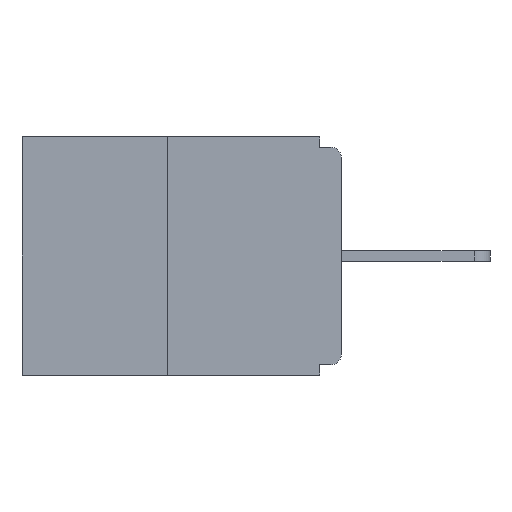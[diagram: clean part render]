
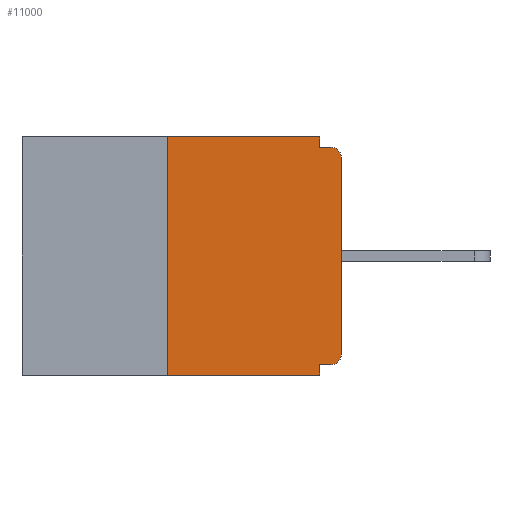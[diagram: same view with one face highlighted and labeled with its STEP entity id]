
A CAD part, left-side view. The second image highlights one B-rep face of the part: STEP entity #11000.
In plain terms, the highlighted planar face has unit normal (-1, 0, 0).
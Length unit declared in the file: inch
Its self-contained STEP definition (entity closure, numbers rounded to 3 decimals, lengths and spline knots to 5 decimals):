
#33 = ORIENTED_EDGE ( 'NONE', *, *, #8551, .F. ) ;
#312 = VERTEX_POINT ( 'NONE', #10353 ) ;
#502 = ORIENTED_EDGE ( 'NONE', *, *, #8499, .T. ) ;
#635 = CARTESIAN_POINT ( 'NONE',  ( 0., 0.031, 0. ) ) ;
#691 = ORIENTED_EDGE ( 'NONE', *, *, #5160, .F. ) ;
#935 = VERTEX_POINT ( 'NONE', #10460 ) ;
#1058 = VERTEX_POINT ( 'NONE', #6445 ) ;
#1236 = ORIENTED_EDGE ( 'NONE', *, *, #5236, .T. ) ;
#2130 = VECTOR ( 'NONE', #8110, 39.37008 ) ;
#2298 = CARTESIAN_POINT ( 'NONE',  ( 0., 0.25, 0. ) ) ;
#2444 = VERTEX_POINT ( 'NONE', #6638 ) ;
#2843 = CARTESIAN_POINT ( 'NONE',  ( 0., 0., -0.313 ) ) ;
#3059 = EDGE_LOOP ( 'NONE', ( #9164, #7493, #502, #33, #8696, #8607, #10615, #1236, #691, #9715 ) ) ;
#3133 = VERTEX_POINT ( 'NONE', #9784 ) ;
#3375 = FACE_OUTER_BOUND ( 'NONE', #3059, .T. ) ;
#3427 = VERTEX_POINT ( 'NONE', #2843 ) ;
#3431 = VERTEX_POINT ( 'NONE', #2298 ) ;
#3560 = EDGE_CURVE ( 'NONE', #3431, #7484, #9764, .T. ) ;
#3712 = LINE ( 'NONE', #10424, #4056 ) ;
#4029 = DIRECTION ( 'NONE',  ( 1., 0., 0. ) ) ;
#4056 = VECTOR ( 'NONE', #10441, 39.37008 ) ;
#4500 = VERTEX_POINT ( 'NONE', #4963 ) ;
#4961 = EDGE_CURVE ( 'NONE', #3427, #935, #11020, .T. ) ;
#4963 = CARTESIAN_POINT ( 'NONE',  ( 0., 0.25, -0.343 ) ) ;
#5100 = EDGE_CURVE ( 'NONE', #8013, #3133, #3712, .T. ) ;
#5160 = EDGE_CURVE ( 'NONE', #312, #1058, #5607, .T. ) ;
#5177 = EDGE_CURVE ( 'NONE', #8013, #3427, #7518, .T. ) ;
#5228 = VECTOR ( 'NONE', #8587, 39.37008 ) ;
#5236 = EDGE_CURVE ( 'NONE', #935, #1058, #7266, .T. ) ;
#5477 = LINE ( 'NONE', #8772, #5228 ) ;
#5510 = AXIS2_PLACEMENT_3D ( 'NONE', #7427, #4029, #9884 ) ;
#5607 = LINE ( 'NONE', #10196, #9704 ) ;
#5889 = CARTESIAN_POINT ( 'NONE',  ( 0., 0.015, -0.328 ) ) ;
#6445 = CARTESIAN_POINT ( 'NONE',  ( 0., 0.015, -0.015 ) ) ;
#6638 = CARTESIAN_POINT ( 'NONE',  ( 0., 0.031, -0.343 ) ) ;
#7266 = CIRCLE ( 'NONE', #10380, 0.015 ) ;
#7394 = VECTOR ( 'NONE', #8279, 39.37008 ) ;
#7427 = CARTESIAN_POINT ( 'NONE',  ( 0., 0.46, 0. ) ) ;
#7484 = VERTEX_POINT ( 'NONE', #635 ) ;
#7493 = ORIENTED_EDGE ( 'NONE', *, *, #8468, .F. ) ;
#7518 = CIRCLE ( 'NONE', #10393, 0.015 ) ;
#7664 = LINE ( 'NONE', #8174, #2130 ) ;
#7919 = LINE ( 'NONE', #9093, #11351 ) ;
#8013 = VERTEX_POINT ( 'NONE', #5889 ) ;
#8110 = DIRECTION ( 'NONE',  ( 0., 0., -1. ) ) ;
#8174 = CARTESIAN_POINT ( 'NONE',  ( 0., 0.031, 0. ) ) ;
#8259 = CARTESIAN_POINT ( 'NONE',  ( 0., 0.031, -0.343 ) ) ;
#8279 = DIRECTION ( 'NONE',  ( 0., 0., -1. ) ) ;
#8468 = EDGE_CURVE ( 'NONE', #4500, #3431, #7919, .T. ) ;
#8499 = EDGE_CURVE ( 'NONE', #4500, #2444, #5477, .T. ) ;
#8551 = EDGE_CURVE ( 'NONE', #3133, #2444, #9348, .T. ) ;
#8552 = EDGE_CURVE ( 'NONE', #7484, #312, #7664, .T. ) ;
#8587 = DIRECTION ( 'NONE',  ( 0., -1., 0. ) ) ;
#8607 = ORIENTED_EDGE ( 'NONE', *, *, #5177, .T. ) ;
#8696 = ORIENTED_EDGE ( 'NONE', *, *, #5100, .F. ) ;
#8772 = CARTESIAN_POINT ( 'NONE',  ( 0., 0.46, -0.343 ) ) ;
#9093 = CARTESIAN_POINT ( 'NONE',  ( 0., 0.25, 0. ) ) ;
#9115 = PLANE ( 'NONE',  #5510 ) ;
#9122 = DIRECTION ( 'NONE',  ( 0., 0., 1. ) ) ;
#9164 = ORIENTED_EDGE ( 'NONE', *, *, #3560, .F. ) ;
#9348 = LINE ( 'NONE', #8259, #7394 ) ;
#9523 = VECTOR ( 'NONE', #10471, 39.37008 ) ;
#9614 = DIRECTION ( 'NONE',  ( 0., 0., -1. ) ) ;
#9628 = DIRECTION ( 'NONE',  ( -1., 0., 0. ) ) ;
#9639 = CARTESIAN_POINT ( 'NONE',  ( 0., 0.015, -0.03 ) ) ;
#9704 = VECTOR ( 'NONE', #10177, 39.37008 ) ;
#9715 = ORIENTED_EDGE ( 'NONE', *, *, #8552, .F. ) ;
#9764 = LINE ( 'NONE', #10487, #9523 ) ;
#9784 = CARTESIAN_POINT ( 'NONE',  ( 0., 0.031, -0.328 ) ) ;
#9834 = VECTOR ( 'NONE', #10932, 39.37008 ) ;
#9884 = DIRECTION ( 'NONE',  ( 0., 0., -1. ) ) ;
#9910 = DIRECTION ( 'NONE',  ( 0., 0., -1. ) ) ;
#9929 = DIRECTION ( 'NONE',  ( -1., 0., 0. ) ) ;
#9940 = CARTESIAN_POINT ( 'NONE',  ( 0., 0.015, -0.313 ) ) ;
#10177 = DIRECTION ( 'NONE',  ( 0., -1., 0. ) ) ;
#10196 = CARTESIAN_POINT ( 'NONE',  ( 0., 0., -0.015 ) ) ;
#10353 = CARTESIAN_POINT ( 'NONE',  ( 0., 0.031, -0.015 ) ) ;
#10380 = AXIS2_PLACEMENT_3D ( 'NONE', #9639, #9628, #9614 ) ;
#10393 = AXIS2_PLACEMENT_3D ( 'NONE', #9940, #9929, #9910 ) ;
#10424 = CARTESIAN_POINT ( 'NONE',  ( 0., 0., -0.328 ) ) ;
#10441 = DIRECTION ( 'NONE',  ( 0., 1., 0. ) ) ;
#10460 = CARTESIAN_POINT ( 'NONE',  ( 0., 0., -0.03 ) ) ;
#10471 = DIRECTION ( 'NONE',  ( 0., -1., 0. ) ) ;
#10487 = CARTESIAN_POINT ( 'NONE',  ( 0., 0.46, 0. ) ) ;
#10615 = ORIENTED_EDGE ( 'NONE', *, *, #4961, .T. ) ;
#10932 = DIRECTION ( 'NONE',  ( 0., 0., 1. ) ) ;
#10944 = CARTESIAN_POINT ( 'NONE',  ( 0., 0., 0. ) ) ;
#11000 = ADVANCED_FACE ( 'NONE', ( #3375 ), #9115, .F. ) ;
#11020 = LINE ( 'NONE', #10944, #9834 ) ;
#11351 = VECTOR ( 'NONE', #9122, 39.37008 ) ;
